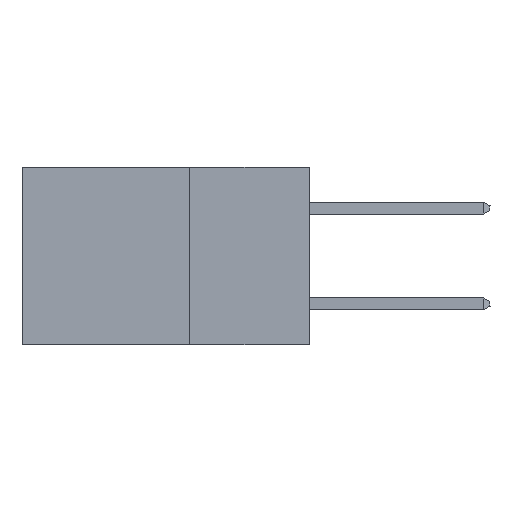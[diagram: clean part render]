
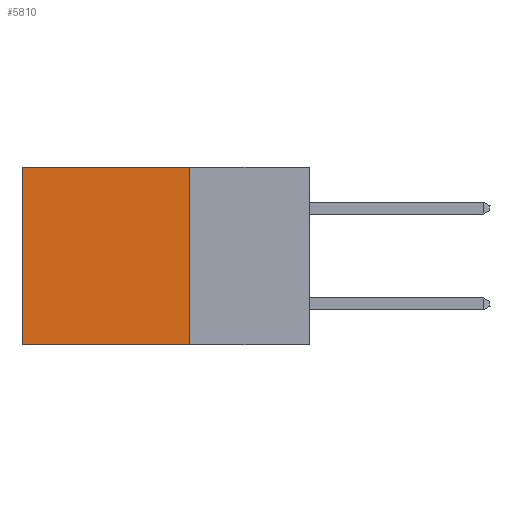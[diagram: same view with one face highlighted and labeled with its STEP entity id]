
A CAD part, left-side view. The second image highlights one B-rep face of the part: STEP entity #5810.
In plain terms, the highlighted planar face has unit normal (-1, 0, 0).
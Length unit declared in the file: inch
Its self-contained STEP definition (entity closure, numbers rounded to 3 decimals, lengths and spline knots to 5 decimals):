
#605 = CARTESIAN_POINT ( 'NONE',  ( 0.2875, 0.6, 0. ) ) ;
#862 = CARTESIAN_POINT ( 'NONE',  ( 0.2875, 0.25, 0. ) ) ;
#2890 = VERTEX_POINT ( 'NONE', #16858 ) ;
#3057 = ORIENTED_EDGE ( 'NONE', *, *, #13706, .T. ) ;
#3264 = CARTESIAN_POINT ( 'NONE',  ( 0.2875, 0.25, -0.37 ) ) ;
#3558 = VERTEX_POINT ( 'NONE', #8126 ) ;
#3960 = AXIS2_PLACEMENT_3D ( 'NONE', #862, #23218, #10113 ) ;
#4960 = DIRECTION ( 'NONE',  ( 0., 1., 0. ) ) ;
#5810 = ADVANCED_FACE ( 'NONE', ( #16418 ), #11388, .F. ) ;
#5990 = ORIENTED_EDGE ( 'NONE', *, *, #19573, .F. ) ;
#7356 = EDGE_LOOP ( 'NONE', ( #10989, #5990, #14122, #3057 ) ) ;
#7433 = VECTOR ( 'NONE', #26320, 39.37008 ) ;
#7449 = LINE ( 'NONE', #15929, #17729 ) ;
#8126 = CARTESIAN_POINT ( 'NONE',  ( 0.2875, 0.25, 0. ) ) ;
#9738 = LINE ( 'NONE', #605, #11808 ) ;
#10113 = DIRECTION ( 'NONE',  ( 0., 0., -1. ) ) ;
#10949 = EDGE_CURVE ( 'NONE', #3558, #11217, #21823, .T. ) ;
#10989 = ORIENTED_EDGE ( 'NONE', *, *, #22649, .T. ) ;
#11217 = VERTEX_POINT ( 'NONE', #22770 ) ;
#11388 = PLANE ( 'NONE',  #3960 ) ;
#11808 = VECTOR ( 'NONE', #26911, 39.37008 ) ;
#12924 = CARTESIAN_POINT ( 'NONE',  ( 0.2875, 0.25, 0. ) ) ;
#13706 = EDGE_CURVE ( 'NONE', #3558, #2890, #7449, .T. ) ;
#14122 = ORIENTED_EDGE ( 'NONE', *, *, #10949, .F. ) ;
#14219 = DIRECTION ( 'NONE',  ( 0., 1., 0. ) ) ;
#15929 = CARTESIAN_POINT ( 'NONE',  ( 0.2875, 0.25, 0. ) ) ;
#16418 = FACE_OUTER_BOUND ( 'NONE', #7356, .T. ) ;
#16858 = CARTESIAN_POINT ( 'NONE',  ( 0.2875, 0.6, 0. ) ) ;
#17131 = VECTOR ( 'NONE', #14219, 39.37008 ) ;
#17729 = VECTOR ( 'NONE', #4960, 39.37008 ) ;
#19573 = EDGE_CURVE ( 'NONE', #11217, #23194, #24978, .T. ) ;
#19639 = CARTESIAN_POINT ( 'NONE',  ( 0.2875, 0.6, -0.37 ) ) ;
#21823 = LINE ( 'NONE', #12924, #7433 ) ;
#22649 = EDGE_CURVE ( 'NONE', #2890, #23194, #9738, .T. ) ;
#22770 = CARTESIAN_POINT ( 'NONE',  ( 0.2875, 0.25, -0.37 ) ) ;
#23194 = VERTEX_POINT ( 'NONE', #19639 ) ;
#23218 = DIRECTION ( 'NONE',  ( 1., 0., 0. ) ) ;
#24978 = LINE ( 'NONE', #3264, #17131 ) ;
#26320 = DIRECTION ( 'NONE',  ( 0., 0., -1. ) ) ;
#26911 = DIRECTION ( 'NONE',  ( 0., 0., -1. ) ) ;
